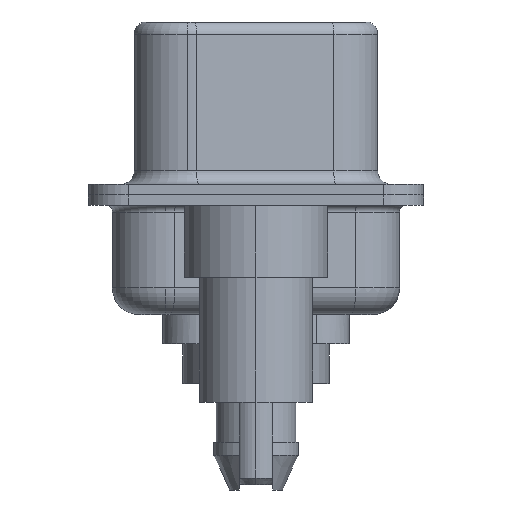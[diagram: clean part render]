
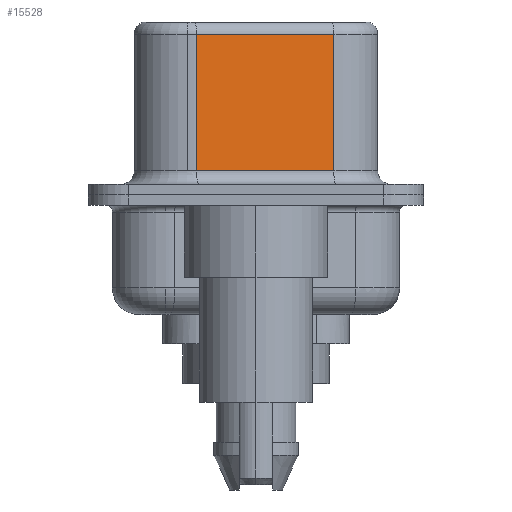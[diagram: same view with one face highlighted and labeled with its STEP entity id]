
A CAD part, left-side view. The second image highlights one B-rep face of the part: STEP entity #15528.
In plain terms, the highlighted planar face has unit normal (-0.985, -0.174, 0).
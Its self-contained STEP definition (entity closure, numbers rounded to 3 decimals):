
#289 = EDGE_CURVE ( 'NONE', #15567, #17517, #17667, .T. ) ;
#1608 = CARTESIAN_POINT ( 'NONE',  ( 4.565, -2.927, 6.52 ) ) ;
#1673 = FACE_OUTER_BOUND ( 'NONE', #8498, .T. ) ;
#1690 = EDGE_CURVE ( 'NONE', #17517, #2933, #11094, .T. ) ;
#2933 = VERTEX_POINT ( 'NONE', #11581 ) ;
#3766 = ORIENTED_EDGE ( 'NONE', *, *, #289, .T. ) ;
#5661 = EDGE_CURVE ( 'NONE', #15567, #12282, #8348, .T. ) ;
#6900 = VECTOR ( 'NONE', #16662, 1000. ) ;
#7154 = CARTESIAN_POINT ( 'NONE',  ( 4.565, -2.927, 0.9 ) ) ;
#7939 = ORIENTED_EDGE ( 'NONE', *, *, #14539, .T. ) ;
#8051 = DIRECTION ( 'NONE',  ( 0.985, 0.174, 0. ) ) ;
#8281 = CARTESIAN_POINT ( 'NONE',  ( 4.565, -2.927, 6.52 ) ) ;
#8348 = LINE ( 'NONE', #8281, #19795 ) ;
#8498 = EDGE_LOOP ( 'NONE', ( #9410, #3766, #16069, #7939 ) ) ;
#9410 = ORIENTED_EDGE ( 'NONE', *, *, #5661, .F. ) ;
#10124 = CARTESIAN_POINT ( 'NONE',  ( 4.565, -2.927, 6.02 ) ) ;
#10936 = LINE ( 'NONE', #7154, #15538 ) ;
#11094 = LINE ( 'NONE', #15122, #6900 ) ;
#11368 = DIRECTION ( 'NONE',  ( 0., 0., -1. ) ) ;
#11581 = CARTESIAN_POINT ( 'NONE',  ( 3.655, 2.233, 0.9 ) ) ;
#12282 = VERTEX_POINT ( 'NONE', #18580 ) ;
#14398 = CARTESIAN_POINT ( 'NONE',  ( 4.565, -2.927, 6.02 ) ) ;
#14539 = EDGE_CURVE ( 'NONE', #2933, #12282, #10936, .T. ) ;
#15122 = CARTESIAN_POINT ( 'NONE',  ( 3.655, 2.233, 6.52 ) ) ;
#15528 = ADVANCED_FACE ( 'NONE', ( #1673 ), #17362, .F. ) ;
#15538 = VECTOR ( 'NONE', #19577, 1000. ) ;
#15567 = VERTEX_POINT ( 'NONE', #14398 ) ;
#16069 = ORIENTED_EDGE ( 'NONE', *, *, #1690, .T. ) ;
#16662 = DIRECTION ( 'NONE',  ( 0., 0., -1. ) ) ;
#17362 = PLANE ( 'NONE',  #17633 ) ;
#17517 = VERTEX_POINT ( 'NONE', #18847 ) ;
#17633 = AXIS2_PLACEMENT_3D ( 'NONE', #1608, #8051, #18942 ) ;
#17667 = LINE ( 'NONE', #10124, #18153 ) ;
#18153 = VECTOR ( 'NONE', #18702, 1000. ) ;
#18580 = CARTESIAN_POINT ( 'NONE',  ( 4.565, -2.927, 0.9 ) ) ;
#18702 = DIRECTION ( 'NONE',  ( -0.174, 0.985, 0. ) ) ;
#18847 = CARTESIAN_POINT ( 'NONE',  ( 3.655, 2.233, 6.02 ) ) ;
#18942 = DIRECTION ( 'NONE',  ( -0.174, 0.985, 0. ) ) ;
#19577 = DIRECTION ( 'NONE',  ( 0.174, -0.985, 0. ) ) ;
#19795 = VECTOR ( 'NONE', #11368, 1000. ) ;
